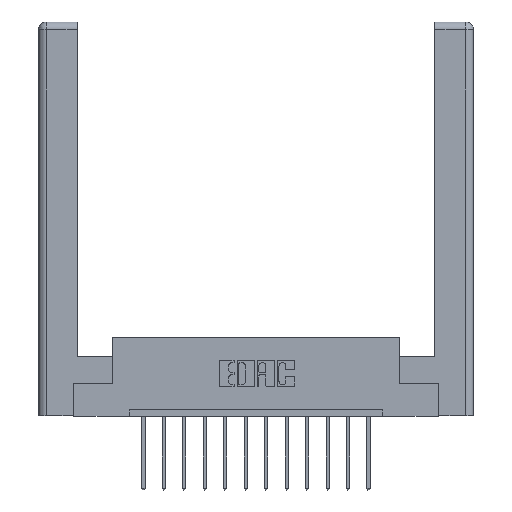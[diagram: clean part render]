
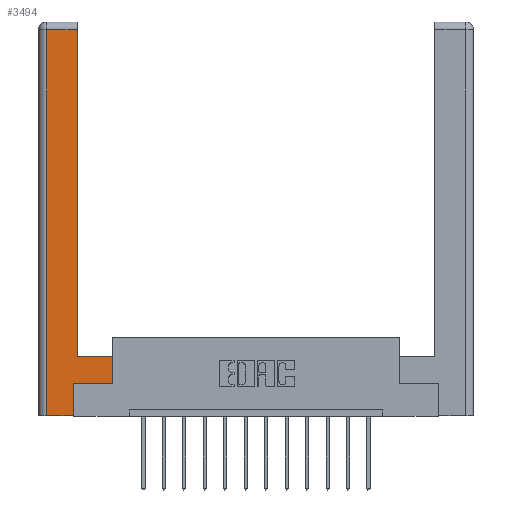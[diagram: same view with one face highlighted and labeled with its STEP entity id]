
A CAD part, top view. The second image highlights one B-rep face of the part: STEP entity #3494.
In plain terms, the highlighted planar face has unit normal (0, 0, 1).
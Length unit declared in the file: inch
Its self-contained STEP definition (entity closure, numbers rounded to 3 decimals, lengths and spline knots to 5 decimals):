
#248 = LINE ( 'NONE', #8767, #6251 ) ;
#416 = VECTOR ( 'NONE', #3197, 39.37008 ) ;
#490 = EDGE_CURVE ( 'NONE', #10952, #4249, #7041, .T. ) ;
#579 = CARTESIAN_POINT ( 'NONE',  ( 0.565, 0.45, 0. ) ) ;
#980 = VERTEX_POINT ( 'NONE', #13996 ) ;
#1261 = VERTEX_POINT ( 'NONE', #2872 ) ;
#1291 = EDGE_CURVE ( 'NONE', #1261, #12622, #13129, .T. ) ;
#1346 = EDGE_CURVE ( 'NONE', #13637, #980, #5693, .T. ) ;
#1751 = LINE ( 'NONE', #3528, #14034 ) ;
#1788 = EDGE_CURVE ( 'NONE', #980, #10952, #248, .T. ) ;
#2141 = ORIENTED_EDGE ( 'NONE', *, *, #490, .T. ) ;
#2617 = EDGE_CURVE ( 'NONE', #12622, #13461, #8467, .T. ) ;
#2634 = DIRECTION ( 'NONE',  ( -1., 0., 0. ) ) ;
#2872 = CARTESIAN_POINT ( 'NONE',  ( 0.265, 0.245, 0. ) ) ;
#2986 = ORIENTED_EDGE ( 'NONE', *, *, #13924, .T. ) ;
#3004 = VECTOR ( 'NONE', #11269, 39.37008 ) ;
#3197 = DIRECTION ( 'NONE',  ( 0., 1., 0. ) ) ;
#3494 = ADVANCED_FACE ( 'NONE', ( #6389 ), #7386, .F. ) ;
#3528 = CARTESIAN_POINT ( 'NONE',  ( 0.265, 0., 0. ) ) ;
#3676 = ORIENTED_EDGE ( 'NONE', *, *, #11854, .T. ) ;
#4249 = VERTEX_POINT ( 'NONE', #10423 ) ;
#4357 = CARTESIAN_POINT ( 'NONE',  ( 0.565, 0.245, 0. ) ) ;
#4530 = CARTESIAN_POINT ( 'NONE',  ( 0.565, 0.45, 0. ) ) ;
#4631 = EDGE_CURVE ( 'NONE', #13461, #13637, #11531, .T. ) ;
#4789 = EDGE_LOOP ( 'NONE', ( #10387, #5221, #2141, #2986, #3676, #11555, #10734, #9148 ) ) ;
#4851 = CARTESIAN_POINT ( 'NONE',  ( 0.265, 0.245, 0. ) ) ;
#4916 = DIRECTION ( 'NONE',  ( 0., 0., -1. ) ) ;
#5221 = ORIENTED_EDGE ( 'NONE', *, *, #1788, .T. ) ;
#5240 = CARTESIAN_POINT ( 'NONE',  ( 0.565, 0.245, 0. ) ) ;
#5312 = VECTOR ( 'NONE', #7840, 39.37008 ) ;
#5355 = VERTEX_POINT ( 'NONE', #11339 ) ;
#5693 = LINE ( 'NONE', #11414, #7579 ) ;
#6251 = VECTOR ( 'NONE', #11011, 39.37008 ) ;
#6389 = FACE_OUTER_BOUND ( 'NONE', #4789, .T. ) ;
#6411 = CARTESIAN_POINT ( 'NONE',  ( 0.0615, 2.94, 0. ) ) ;
#7041 = LINE ( 'NONE', #14941, #12958 ) ;
#7386 = PLANE ( 'NONE',  #14324 ) ;
#7579 = VECTOR ( 'NONE', #8960, 39.37008 ) ;
#7840 = DIRECTION ( 'NONE',  ( 1., 0., 0. ) ) ;
#8467 = LINE ( 'NONE', #4530, #416 ) ;
#8767 = CARTESIAN_POINT ( 'NONE',  ( 0.0615, 2.94, 0. ) ) ;
#8915 = CARTESIAN_POINT ( 'NONE',  ( 0.295, 0.45, 0. ) ) ;
#8960 = DIRECTION ( 'NONE',  ( 0., 1., 0. ) ) ;
#9148 = ORIENTED_EDGE ( 'NONE', *, *, #4631, .T. ) ;
#9538 = DIRECTION ( 'NONE',  ( 0., 1., 0. ) ) ;
#9670 = DIRECTION ( 'NONE',  ( 1., 0., 0. ) ) ;
#9849 = CARTESIAN_POINT ( 'NONE',  ( 0., 0., 0. ) ) ;
#10181 = DIRECTION ( 'NONE',  ( 0., -1., 0. ) ) ;
#10387 = ORIENTED_EDGE ( 'NONE', *, *, #1346, .T. ) ;
#10423 = CARTESIAN_POINT ( 'NONE',  ( 0.0615, 0., 0. ) ) ;
#10734 = ORIENTED_EDGE ( 'NONE', *, *, #2617, .T. ) ;
#10952 = VERTEX_POINT ( 'NONE', #6411 ) ;
#11011 = DIRECTION ( 'NONE',  ( -1., 0., 0. ) ) ;
#11269 = DIRECTION ( 'NONE',  ( -1., 0., 0. ) ) ;
#11339 = CARTESIAN_POINT ( 'NONE',  ( 0.265, 0., 0. ) ) ;
#11414 = CARTESIAN_POINT ( 'NONE',  ( 0.295, 3., 0. ) ) ;
#11531 = LINE ( 'NONE', #8915, #3004 ) ;
#11555 = ORIENTED_EDGE ( 'NONE', *, *, #1291, .T. ) ;
#11854 = EDGE_CURVE ( 'NONE', #5355, #1261, #12795, .T. ) ;
#12622 = VERTEX_POINT ( 'NONE', #5240 ) ;
#12795 = LINE ( 'NONE', #4851, #14677 ) ;
#12958 = VECTOR ( 'NONE', #10181, 39.37008 ) ;
#13129 = LINE ( 'NONE', #4357, #5312 ) ;
#13461 = VERTEX_POINT ( 'NONE', #579 ) ;
#13637 = VERTEX_POINT ( 'NONE', #15469 ) ;
#13924 = EDGE_CURVE ( 'NONE', #4249, #5355, #1751, .T. ) ;
#13996 = CARTESIAN_POINT ( 'NONE',  ( 0.295, 2.94, 0. ) ) ;
#14034 = VECTOR ( 'NONE', #9670, 39.37008 ) ;
#14324 = AXIS2_PLACEMENT_3D ( 'NONE', #9849, #4916, #2634 ) ;
#14677 = VECTOR ( 'NONE', #9538, 39.37008 ) ;
#14941 = CARTESIAN_POINT ( 'NONE',  ( 0.0615, 0., 0. ) ) ;
#15469 = CARTESIAN_POINT ( 'NONE',  ( 0.295, 0.45, 0. ) ) ;
